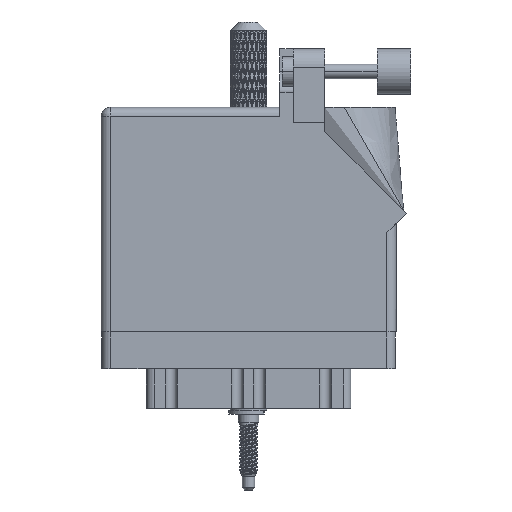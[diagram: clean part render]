
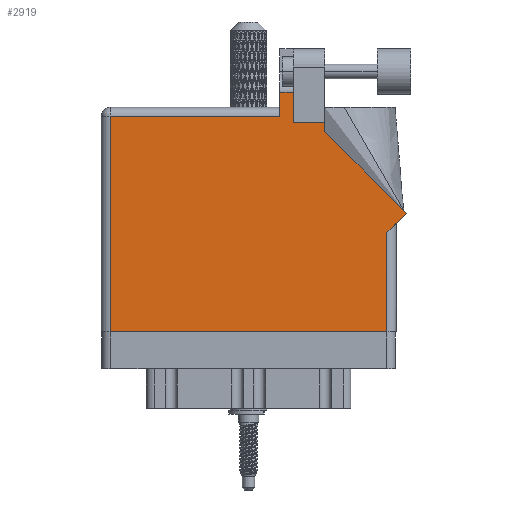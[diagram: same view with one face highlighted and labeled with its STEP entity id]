
A CAD part, front view. The second image highlights one B-rep face of the part: STEP entity #2919.
In plain terms, the highlighted face is planar.
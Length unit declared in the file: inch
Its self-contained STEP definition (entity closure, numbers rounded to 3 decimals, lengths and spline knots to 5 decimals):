
#1317 = CARTESIAN_POINT ( 'NONE',  ( 0., 1.53, 0. ) ) ;
#1843 = VECTOR ( 'NONE', #51652, 39.37008 ) ;
#2919 = ADVANCED_FACE ( 'NONE', ( #9772 ), #68075, .F. ) ;
#3736 = CARTESIAN_POINT ( 'NONE',  ( 1.311, 1.6315, 0. ) ) ;
#5228 = VECTOR ( 'NONE', #11200, 39.37008 ) ;
#5312 = VERTEX_POINT ( 'NONE', #34963 ) ;
#6064 = LINE ( 'NONE', #104140, #83623 ) ;
#7741 = VECTOR ( 'NONE', #79419, 39.37008 ) ;
#8624 = CARTESIAN_POINT ( 'NONE',  ( 1.311, 1.43, 0. ) ) ;
#9338 = ORIENTED_EDGE ( 'NONE', *, *, #57498, .T. ) ;
#9772 = FACE_OUTER_BOUND ( 'NONE', #64182, .T. ) ;
#10069 = ORIENTED_EDGE ( 'NONE', *, *, #18560, .T. ) ;
#10926 = VERTEX_POINT ( 'NONE', #85780 ) ;
#11200 = DIRECTION ( 'NONE',  ( -1., 0., 0. ) ) ;
#11630 = CARTESIAN_POINT ( 'NONE',  ( 1.948, 0.675, 0. ) ) ;
#13466 = DIRECTION ( 'NONE',  ( 1., 0., 0. ) ) ;
#14670 = VERTEX_POINT ( 'NONE', #93248 ) ;
#18560 = EDGE_CURVE ( 'NONE', #5312, #10926, #82800, .T. ) ;
#19850 = DIRECTION ( 'NONE',  ( 0., 0., -1. ) ) ;
#20279 = LINE ( 'NONE', #61622, #77243 ) ;
#21647 = LINE ( 'NONE', #61934, #39124 ) ;
#23148 = VERTEX_POINT ( 'NONE', #67019 ) ;
#24057 = DIRECTION ( 'NONE',  ( 0., -1., 0. ) ) ;
#25832 = DIRECTION ( 'NONE',  ( 0.707, 0.707, 0. ) ) ;
#26754 = DIRECTION ( 'NONE',  ( -1., 0., 0. ) ) ;
#27236 = VERTEX_POINT ( 'NONE', #49270 ) ;
#29022 = CARTESIAN_POINT ( 'NONE',  ( 1.311, 1.43, 0. ) ) ;
#30020 = VECTOR ( 'NONE', #59260, 39.37008 ) ;
#32982 = EDGE_CURVE ( 'NONE', #77961, #23148, #66078, .T. ) ;
#34478 = CARTESIAN_POINT ( 'NONE',  ( 1.524, 1.36442, 0. ) ) ;
#34963 = CARTESIAN_POINT ( 'NONE',  ( 1.217, 1.468, 0. ) ) ;
#35909 = CARTESIAN_POINT ( 'NONE',  ( 1.64177, 1.6315, 0. ) ) ;
#39124 = VECTOR ( 'NONE', #95336, 39.37008 ) ;
#39495 = LINE ( 'NONE', #71828, #88935 ) ;
#40006 = DIRECTION ( 'NONE',  ( 0., 1., 0. ) ) ;
#42406 = EDGE_CURVE ( 'NONE', #70087, #27236, #6064, .T. ) ;
#42629 = CARTESIAN_POINT ( 'NONE',  ( 0.062, 0., 0. ) ) ;
#43892 = EDGE_CURVE ( 'NONE', #23148, #66039, #21647, .T. ) ;
#46599 = ORIENTED_EDGE ( 'NONE', *, *, #42406, .T. ) ;
#48454 = CARTESIAN_POINT ( 'NONE',  ( 1.217, 1.53, 0. ) ) ;
#48492 = ORIENTED_EDGE ( 'NONE', *, *, #96506, .T. ) ;
#48600 = ORIENTED_EDGE ( 'NONE', *, *, #55930, .T. ) ;
#49270 = CARTESIAN_POINT ( 'NONE',  ( 1.948, 0., 0. ) ) ;
#51652 = DIRECTION ( 'NONE',  ( 0., 1., 0. ) ) ;
#51907 = EDGE_CURVE ( 'NONE', #27236, #77961, #39495, .T. ) ;
#53028 = AXIS2_PLACEMENT_3D ( 'NONE', #1317, #19850, #26754 ) ;
#55234 = ORIENTED_EDGE ( 'NONE', *, *, #83523, .T. ) ;
#55724 = EDGE_CURVE ( 'NONE', #10926, #70087, #20279, .T. ) ;
#55930 = EDGE_CURVE ( 'NONE', #76895, #86252, #77273, .T. ) ;
#57498 = EDGE_CURVE ( 'NONE', #86252, #14670, #68735, .T. ) ;
#58966 = CARTESIAN_POINT ( 'NONE',  ( 0., 1.468, 0. ) ) ;
#59260 = DIRECTION ( 'NONE',  ( -1., 0., 0. ) ) ;
#59548 = ORIENTED_EDGE ( 'NONE', *, *, #43892, .T. ) ;
#61357 = DIRECTION ( 'NONE',  ( 0., 1., 0. ) ) ;
#61622 = CARTESIAN_POINT ( 'NONE',  ( 0.062, 0., 0. ) ) ;
#61895 = ORIENTED_EDGE ( 'NONE', *, *, #85856, .T. ) ;
#61934 = CARTESIAN_POINT ( 'NONE',  ( 2.08071, 0.80771, 0. ) ) ;
#64182 = EDGE_LOOP ( 'NONE', ( #48600, #9338, #61895, #10069, #82490, #46599, #99088, #82230, #59548, #55234, #48492 ) ) ;
#65410 = VECTOR ( 'NONE', #61357, 39.37008 ) ;
#66039 = VERTEX_POINT ( 'NONE', #34478 ) ;
#66078 = LINE ( 'NONE', #98461, #74531 ) ;
#67019 = CARTESIAN_POINT ( 'NONE',  ( 2.08071, 0.80771, 0. ) ) ;
#67390 = CARTESIAN_POINT ( 'NONE',  ( 1.524, 1.43, 0. ) ) ;
#68075 = PLANE ( 'NONE',  #53028 ) ;
#68735 = LINE ( 'NONE', #35909, #30020 ) ;
#70087 = VERTEX_POINT ( 'NONE', #42629 ) ;
#71828 = CARTESIAN_POINT ( 'NONE',  ( 1.948, 0.737, 0. ) ) ;
#74531 = VECTOR ( 'NONE', #25832, 39.37008 ) ;
#76895 = VERTEX_POINT ( 'NONE', #8624 ) ;
#77003 = DIRECTION ( 'NONE',  ( 0., -1., 0. ) ) ;
#77243 = VECTOR ( 'NONE', #77003, 39.37008 ) ;
#77273 = LINE ( 'NONE', #29022, #65410 ) ;
#77961 = VERTEX_POINT ( 'NONE', #11630 ) ;
#79419 = DIRECTION ( 'NONE',  ( -1., 0., 0. ) ) ;
#82230 = ORIENTED_EDGE ( 'NONE', *, *, #32982, .T. ) ;
#82490 = ORIENTED_EDGE ( 'NONE', *, *, #55724, .T. ) ;
#82800 = LINE ( 'NONE', #58966, #5228 ) ;
#83523 = EDGE_CURVE ( 'NONE', #66039, #96226, #91425, .T. ) ;
#83623 = VECTOR ( 'NONE', #13466, 39.37008 ) ;
#85780 = CARTESIAN_POINT ( 'NONE',  ( 0.062, 1.468, 0. ) ) ;
#85856 = EDGE_CURVE ( 'NONE', #14670, #5312, #96710, .T. ) ;
#86252 = VERTEX_POINT ( 'NONE', #3736 ) ;
#88935 = VECTOR ( 'NONE', #40006, 39.37008 ) ;
#91425 = LINE ( 'NONE', #100414, #1843 ) ;
#91712 = VECTOR ( 'NONE', #24057, 39.37008 ) ;
#93248 = CARTESIAN_POINT ( 'NONE',  ( 1.217, 1.6315, 0. ) ) ;
#95336 = DIRECTION ( 'NONE',  ( -0.707, 0.707, 0. ) ) ;
#95853 = CARTESIAN_POINT ( 'NONE',  ( 1.524, 1.43, 0. ) ) ;
#96226 = VERTEX_POINT ( 'NONE', #67390 ) ;
#96506 = EDGE_CURVE ( 'NONE', #96226, #76895, #102759, .T. ) ;
#96710 = LINE ( 'NONE', #48454, #91712 ) ;
#98461 = CARTESIAN_POINT ( 'NONE',  ( 2.01, 0.737, 0. ) ) ;
#99088 = ORIENTED_EDGE ( 'NONE', *, *, #51907, .T. ) ;
#100414 = CARTESIAN_POINT ( 'NONE',  ( 1.524, 1.36442, 0. ) ) ;
#102759 = LINE ( 'NONE', #95853, #7741 ) ;
#104140 = CARTESIAN_POINT ( 'NONE',  ( 0., 0., 0. ) ) ;
